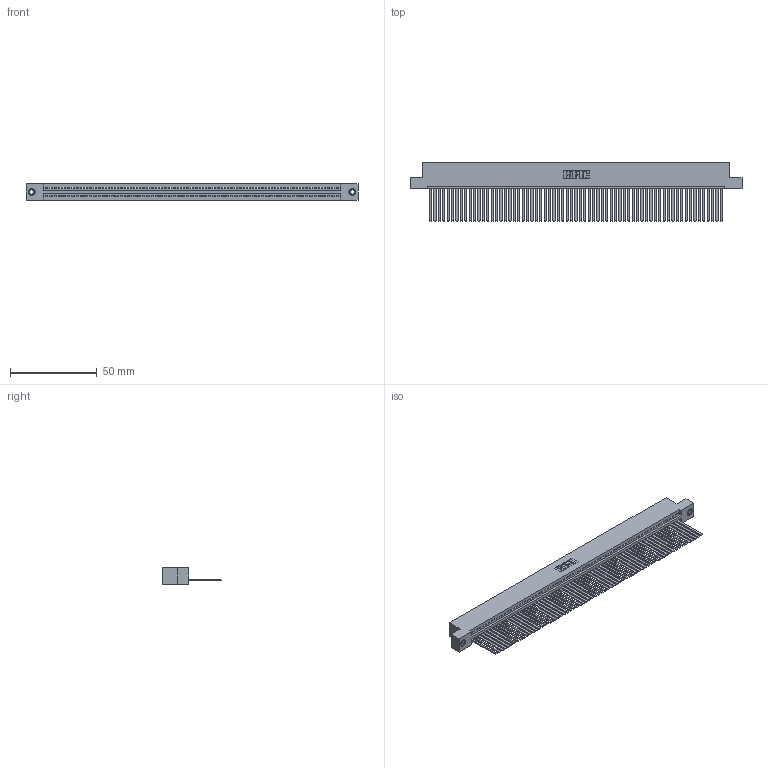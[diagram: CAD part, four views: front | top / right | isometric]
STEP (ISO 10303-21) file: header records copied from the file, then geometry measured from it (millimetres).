
FILE_DESCRIPTION (( 'STEP AP203' ), '1' );
FILE_NAME ('345-067-544-107.STEP', '2019-10-12T02:56:35', ( '' ), ( '' ), 'SwSTEP 2.0', 'SolidWorks 2016', '' );
FILE_SCHEMA (( 'CONFIG_CONTROL_DESIGN' ));
Length unit declared in the file: inch
Products named in the file (4): 345-067-544-107; 345-250-001_345-250-005-103; 345-292-001_345-293-144; 345 Part_Flush Mounting Lugs - 0.156 Dia-TI
Assembly tree (70 placements, depth 2):
  345-067-544-107
    345 Part_Flush Mounting Lugs - 0.156 Dia-TI
    345-292-001_345-293-144  x67
    345-250-001_345-250-005-103  x2
Bounding box: 191.39 x 33.96 x 9.4 mm (x, y, z)
Volume: 19145.5 mm3; surface area: 28144.5 mm2
Topology: 70 solids, 70 shells, 3670 faces, 11063 edges, 7278 vertices
Faces by surface type: plane 2524, cylinder 1130, cone 12, torus 4
Entity records: 48062 total; most frequent: CARTESIAN_POINT 8304, ORIENTED_EDGE 8298, DIRECTION 7241, EDGE_CURVE 4149, LINE 3733, VECTOR 3733, VERTEX_POINT 2760, AXIS2_PLACEMENT_3D 1754
